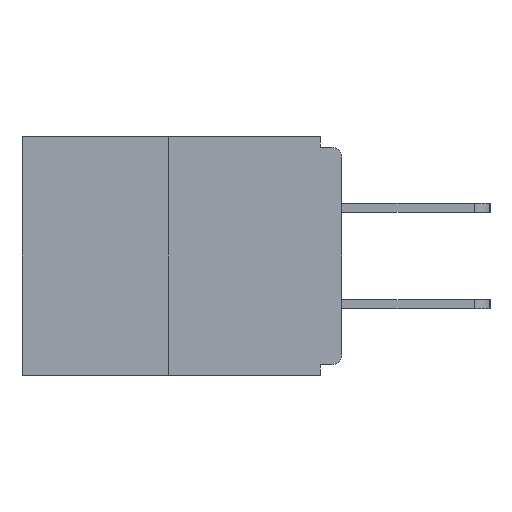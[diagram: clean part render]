
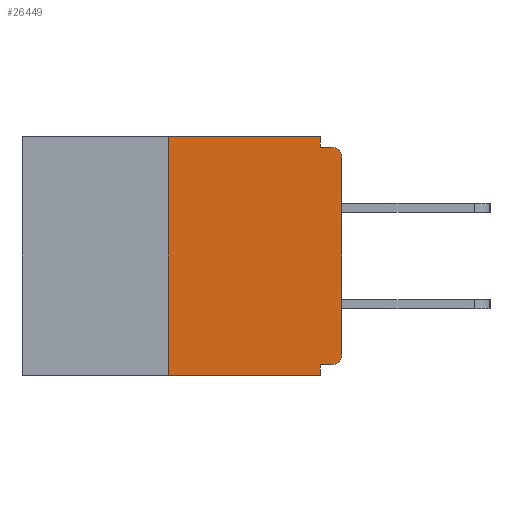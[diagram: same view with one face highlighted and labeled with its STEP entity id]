
A CAD part, left-side view. The second image highlights one B-rep face of the part: STEP entity #26449.
In plain terms, the highlighted planar face has unit normal (-1, 0, 0).
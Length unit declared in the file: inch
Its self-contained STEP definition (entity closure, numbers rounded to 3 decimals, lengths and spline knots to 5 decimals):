
#196 = ORIENTED_EDGE ( 'NONE', *, *, #8310, .F. ) ;
#205 = EDGE_LOOP ( 'NONE', ( #16789, #20267, #28044, #20451, #11091, #3591, #2444, #18044, #196, #20623 ) ) ;
#551 = DIRECTION ( 'NONE',  ( 0., 0., 1. ) ) ;
#670 = VERTEX_POINT ( 'NONE', #863 ) ;
#863 = CARTESIAN_POINT ( 'NONE',  ( 0., 0.031, 0. ) ) ;
#1245 = DIRECTION ( 'NONE',  ( -1., 0., 0. ) ) ;
#1435 = DIRECTION ( 'NONE',  ( 0., 0., -1. ) ) ;
#2106 = CARTESIAN_POINT ( 'NONE',  ( 0., 0.031, -0.343 ) ) ;
#2214 = CARTESIAN_POINT ( 'NONE',  ( 0., 0.25, -0.343 ) ) ;
#2444 = ORIENTED_EDGE ( 'NONE', *, *, #18979, .T. ) ;
#2791 = VERTEX_POINT ( 'NONE', #4596 ) ;
#3082 = CARTESIAN_POINT ( 'NONE',  ( 0., 0.25, 0. ) ) ;
#3435 = DIRECTION ( 'NONE',  ( 0., -1., 0. ) ) ;
#3482 = EDGE_CURVE ( 'NONE', #670, #2791, #17739, .T. ) ;
#3591 = ORIENTED_EDGE ( 'NONE', *, *, #7270, .T. ) ;
#3739 = CARTESIAN_POINT ( 'NONE',  ( 0., 0.015, -0.03 ) ) ;
#4006 = CARTESIAN_POINT ( 'NONE',  ( 0., 0.46, 0. ) ) ;
#4596 = CARTESIAN_POINT ( 'NONE',  ( 0., 0.031, -0.015 ) ) ;
#4778 = DIRECTION ( 'NONE',  ( 0., 0., -1. ) ) ;
#4910 = DIRECTION ( 'NONE',  ( 0., 0., -1. ) ) ;
#5014 = LINE ( 'NONE', #19247, #28256 ) ;
#5036 = VECTOR ( 'NONE', #4778, 39.37008 ) ;
#6130 = AXIS2_PLACEMENT_3D ( 'NONE', #3739, #1245, #12321 ) ;
#6433 = VECTOR ( 'NONE', #8606, 39.37008 ) ;
#7172 = CARTESIAN_POINT ( 'NONE',  ( 0., 0., 0. ) ) ;
#7270 = EDGE_CURVE ( 'NONE', #22437, #15593, #9232, .T. ) ;
#7352 = EDGE_CURVE ( 'NONE', #12314, #19111, #23210, .T. ) ;
#7597 = VERTEX_POINT ( 'NONE', #8071 ) ;
#8071 = CARTESIAN_POINT ( 'NONE',  ( 0., 0., -0.03 ) ) ;
#8136 = LINE ( 'NONE', #2106, #5036 ) ;
#8310 = EDGE_CURVE ( 'NONE', #2791, #15557, #12904, .T. ) ;
#8364 = VECTOR ( 'NONE', #1435, 39.37008 ) ;
#8414 = DIRECTION ( 'NONE',  ( 0., -1., 0. ) ) ;
#8479 = EDGE_CURVE ( 'NONE', #19111, #670, #15923, .T. ) ;
#8606 = DIRECTION ( 'NONE',  ( 0., -1., 0. ) ) ;
#8900 = EDGE_CURVE ( 'NONE', #22437, #26702, #16574, .T. ) ;
#9232 = CIRCLE ( 'NONE', #14826, 0.015 ) ;
#9268 = DIRECTION ( 'NONE',  ( 0., 0., -1. ) ) ;
#9693 = DIRECTION ( 'NONE',  ( 0., 0., 1. ) ) ;
#10608 = CARTESIAN_POINT ( 'NONE',  ( 0., 0.031, -0.328 ) ) ;
#11091 = ORIENTED_EDGE ( 'NONE', *, *, #8900, .F. ) ;
#11301 = AXIS2_PLACEMENT_3D ( 'NONE', #20037, #25108, #9268 ) ;
#11847 = VECTOR ( 'NONE', #25998, 39.37008 ) ;
#12314 = VERTEX_POINT ( 'NONE', #2214 ) ;
#12321 = DIRECTION ( 'NONE',  ( 0., 0., -1. ) ) ;
#12904 = LINE ( 'NONE', #25592, #25548 ) ;
#13191 = CARTESIAN_POINT ( 'NONE',  ( 0., 0., -0.328 ) ) ;
#13212 = CIRCLE ( 'NONE', #6130, 0.015 ) ;
#13533 = PLANE ( 'NONE',  #11301 ) ;
#13763 = DIRECTION ( 'NONE',  ( -1., 0., 0. ) ) ;
#13853 = CARTESIAN_POINT ( 'NONE',  ( 0., 0.015, -0.313 ) ) ;
#14633 = CARTESIAN_POINT ( 'NONE',  ( 0., 0.015, -0.328 ) ) ;
#14826 = AXIS2_PLACEMENT_3D ( 'NONE', #13853, #13763, #4910 ) ;
#15557 = VERTEX_POINT ( 'NONE', #28097 ) ;
#15593 = VERTEX_POINT ( 'NONE', #17645 ) ;
#15923 = LINE ( 'NONE', #4006, #6433 ) ;
#16574 = LINE ( 'NONE', #13191, #11847 ) ;
#16607 = EDGE_CURVE ( 'NONE', #26702, #17925, #8136, .T. ) ;
#16789 = ORIENTED_EDGE ( 'NONE', *, *, #8479, .F. ) ;
#17381 = VECTOR ( 'NONE', #9693, 39.37008 ) ;
#17645 = CARTESIAN_POINT ( 'NONE',  ( 0., 0., -0.313 ) ) ;
#17739 = LINE ( 'NONE', #23320, #8364 ) ;
#17925 = VERTEX_POINT ( 'NONE', #18534 ) ;
#18044 = ORIENTED_EDGE ( 'NONE', *, *, #22995, .T. ) ;
#18534 = CARTESIAN_POINT ( 'NONE',  ( 0., 0.031, -0.343 ) ) ;
#18979 = EDGE_CURVE ( 'NONE', #15593, #7597, #21977, .T. ) ;
#19111 = VERTEX_POINT ( 'NONE', #27070 ) ;
#19247 = CARTESIAN_POINT ( 'NONE',  ( 0., 0.46, -0.343 ) ) ;
#20037 = CARTESIAN_POINT ( 'NONE',  ( 0., 0.46, 0. ) ) ;
#20267 = ORIENTED_EDGE ( 'NONE', *, *, #7352, .F. ) ;
#20451 = ORIENTED_EDGE ( 'NONE', *, *, #16607, .F. ) ;
#20623 = ORIENTED_EDGE ( 'NONE', *, *, #3482, .F. ) ;
#21977 = LINE ( 'NONE', #7172, #24392 ) ;
#22437 = VERTEX_POINT ( 'NONE', #14633 ) ;
#22995 = EDGE_CURVE ( 'NONE', #7597, #15557, #13212, .T. ) ;
#23210 = LINE ( 'NONE', #3082, #17381 ) ;
#23320 = CARTESIAN_POINT ( 'NONE',  ( 0., 0.031, 0. ) ) ;
#23462 = FACE_OUTER_BOUND ( 'NONE', #205, .T. ) ;
#23787 = EDGE_CURVE ( 'NONE', #12314, #17925, #5014, .T. ) ;
#24392 = VECTOR ( 'NONE', #551, 39.37008 ) ;
#25108 = DIRECTION ( 'NONE',  ( 1., 0., 0. ) ) ;
#25548 = VECTOR ( 'NONE', #3435, 39.37008 ) ;
#25592 = CARTESIAN_POINT ( 'NONE',  ( 0., 0., -0.015 ) ) ;
#25998 = DIRECTION ( 'NONE',  ( 0., 1., 0. ) ) ;
#26449 = ADVANCED_FACE ( 'NONE', ( #23462 ), #13533, .F. ) ;
#26702 = VERTEX_POINT ( 'NONE', #10608 ) ;
#27070 = CARTESIAN_POINT ( 'NONE',  ( 0., 0.25, 0. ) ) ;
#28044 = ORIENTED_EDGE ( 'NONE', *, *, #23787, .T. ) ;
#28097 = CARTESIAN_POINT ( 'NONE',  ( 0., 0.015, -0.015 ) ) ;
#28256 = VECTOR ( 'NONE', #8414, 39.37008 ) ;
